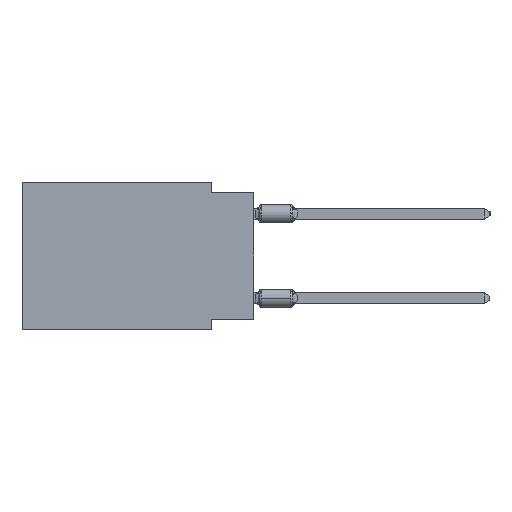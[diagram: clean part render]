
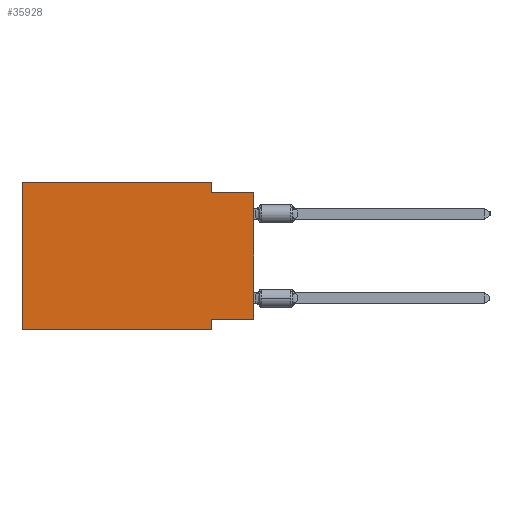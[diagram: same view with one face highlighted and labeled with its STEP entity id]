
A CAD part, left-side view. The second image highlights one B-rep face of the part: STEP entity #35928.
In plain terms, the highlighted planar face has unit normal (-1, 0, 0).
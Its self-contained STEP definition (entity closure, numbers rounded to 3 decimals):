
#1658 = PLANE ( 'NONE',  #6181 ) ;
#2259 = VERTEX_POINT ( 'NONE', #30086 ) ;
#3256 = ORIENTED_EDGE ( 'NONE', *, *, #21316, .F. ) ;
#5895 = VERTEX_POINT ( 'NONE', #9294 ) ;
#6181 = AXIS2_PLACEMENT_3D ( 'NONE', #16853, #11893, #6928 ) ;
#6928 = DIRECTION ( 'NONE',  ( 0., 0., -1. ) ) ;
#8041 = EDGE_CURVE ( 'NONE', #25720, #38384, #19394, .T. ) ;
#8290 = VECTOR ( 'NONE', #43614, 1000. ) ;
#8743 = CARTESIAN_POINT ( 'NONE',  ( 0., 13.97, 0. ) ) ;
#8986 = CARTESIAN_POINT ( 'NONE',  ( 0., 0., -0.635 ) ) ;
#9294 = CARTESIAN_POINT ( 'NONE',  ( 0., 2.54, 0. ) ) ;
#10026 = CARTESIAN_POINT ( 'NONE',  ( 0., 0., -8.255 ) ) ;
#10704 = DIRECTION ( 'NONE',  ( 0., 0., 1. ) ) ;
#11562 = DIRECTION ( 'NONE',  ( 0., 0., -1. ) ) ;
#11893 = DIRECTION ( 'NONE',  ( 1., 0., 0. ) ) ;
#13023 = CARTESIAN_POINT ( 'NONE',  ( 0., 13.97, -8.89 ) ) ;
#13715 = LINE ( 'NONE', #8743, #58755 ) ;
#14403 = DIRECTION ( 'NONE',  ( 0., -1., 0. ) ) ;
#15135 = ORIENTED_EDGE ( 'NONE', *, *, #45512, .T. ) ;
#16853 = CARTESIAN_POINT ( 'NONE',  ( 0., 13.97, 0. ) ) ;
#17073 = EDGE_CURVE ( 'NONE', #25720, #23694, #13715, .T. ) ;
#17256 = DIRECTION ( 'NONE',  ( 0., -1., 0. ) ) ;
#19394 = LINE ( 'NONE', #48280, #8290 ) ;
#21316 = EDGE_CURVE ( 'NONE', #57231, #43558, #41457, .T. ) ;
#23080 = VECTOR ( 'NONE', #52333, 1000. ) ;
#23694 = VERTEX_POINT ( 'NONE', #46439 ) ;
#24418 = EDGE_CURVE ( 'NONE', #5895, #57231, #58464, .T. ) ;
#24457 = VECTOR ( 'NONE', #17256, 1000. ) ;
#24980 = VECTOR ( 'NONE', #11562, 1000. ) ;
#25720 = VERTEX_POINT ( 'NONE', #13023 ) ;
#29035 = ORIENTED_EDGE ( 'NONE', *, *, #56055, .F. ) ;
#29298 = CARTESIAN_POINT ( 'NONE',  ( 0., 13.97, 0. ) ) ;
#29494 = ORIENTED_EDGE ( 'NONE', *, *, #43866, .F. ) ;
#30086 = CARTESIAN_POINT ( 'NONE',  ( 0., 2.54, -8.255 ) ) ;
#32784 = ORIENTED_EDGE ( 'NONE', *, *, #24418, .F. ) ;
#33383 = CARTESIAN_POINT ( 'NONE',  ( 0., 2.54, -8.89 ) ) ;
#33499 = ORIENTED_EDGE ( 'NONE', *, *, #17073, .F. ) ;
#34521 = VECTOR ( 'NONE', #53700, 1000. ) ;
#34755 = CARTESIAN_POINT ( 'NONE',  ( 0., 0., -8.255 ) ) ;
#35928 = ADVANCED_FACE ( 'NONE', ( #48547 ), #1658, .F. ) ;
#36746 = EDGE_LOOP ( 'NONE', ( #15135, #3256, #32784, #29035, #33499, #51363, #49322, #29494 ) ) ;
#37222 = EDGE_CURVE ( 'NONE', #2259, #38384, #38355, .T. ) ;
#38053 = LINE ( 'NONE', #48292, #54473 ) ;
#38355 = LINE ( 'NONE', #33383, #23080 ) ;
#38384 = VERTEX_POINT ( 'NONE', #51416 ) ;
#41457 = LINE ( 'NONE', #50486, #24457 ) ;
#43558 = VERTEX_POINT ( 'NONE', #8986 ) ;
#43614 = DIRECTION ( 'NONE',  ( 0., -1., 0. ) ) ;
#43866 = EDGE_CURVE ( 'NONE', #52965, #2259, #49969, .T. ) ;
#45512 = EDGE_CURVE ( 'NONE', #52965, #43558, #38053, .T. ) ;
#46439 = CARTESIAN_POINT ( 'NONE',  ( 0., 13.97, 0. ) ) ;
#48111 = DIRECTION ( 'NONE',  ( 0., 0., 1. ) ) ;
#48280 = CARTESIAN_POINT ( 'NONE',  ( 0., 13.97, -8.89 ) ) ;
#48292 = CARTESIAN_POINT ( 'NONE',  ( 0., 0., 0. ) ) ;
#48547 = FACE_OUTER_BOUND ( 'NONE', #36746, .T. ) ;
#49322 = ORIENTED_EDGE ( 'NONE', *, *, #37222, .F. ) ;
#49420 = CARTESIAN_POINT ( 'NONE',  ( 0., 2.54, -0.635 ) ) ;
#49969 = LINE ( 'NONE', #34755, #34521 ) ;
#50486 = CARTESIAN_POINT ( 'NONE',  ( 0., 0., -0.635 ) ) ;
#51363 = ORIENTED_EDGE ( 'NONE', *, *, #8041, .T. ) ;
#51416 = CARTESIAN_POINT ( 'NONE',  ( 0., 2.54, -8.89 ) ) ;
#51914 = VECTOR ( 'NONE', #14403, 1000. ) ;
#52333 = DIRECTION ( 'NONE',  ( 0., 0., -1. ) ) ;
#52965 = VERTEX_POINT ( 'NONE', #10026 ) ;
#53700 = DIRECTION ( 'NONE',  ( 0., 1., 0. ) ) ;
#54117 = CARTESIAN_POINT ( 'NONE',  ( 0., 2.54, 0. ) ) ;
#54473 = VECTOR ( 'NONE', #10704, 1000. ) ;
#56055 = EDGE_CURVE ( 'NONE', #23694, #5895, #57560, .T. ) ;
#57231 = VERTEX_POINT ( 'NONE', #49420 ) ;
#57560 = LINE ( 'NONE', #29298, #51914 ) ;
#58464 = LINE ( 'NONE', #54117, #24980 ) ;
#58755 = VECTOR ( 'NONE', #48111, 1000. ) ;
